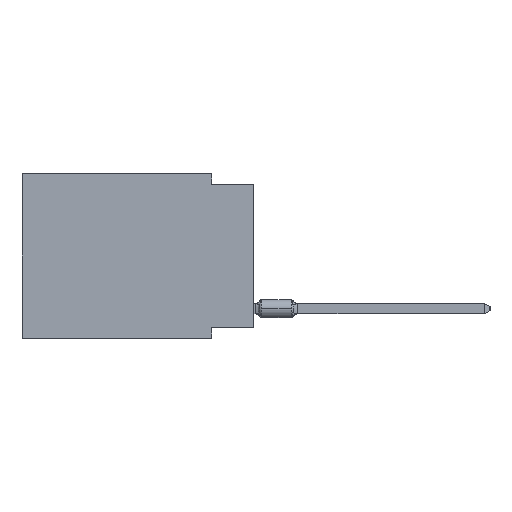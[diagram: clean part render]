
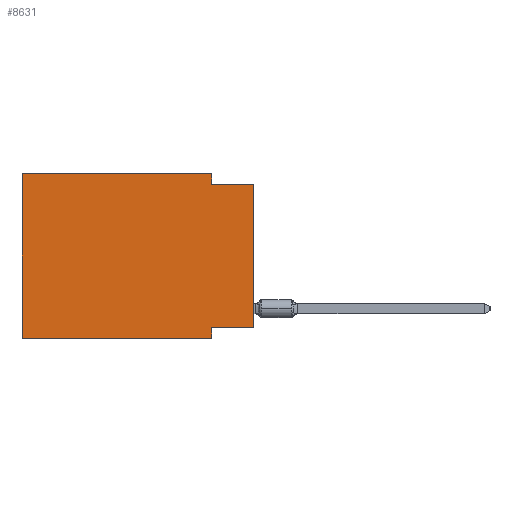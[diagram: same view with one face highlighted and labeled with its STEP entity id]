
A CAD part, left-side view. The second image highlights one B-rep face of the part: STEP entity #8631.
In plain terms, the highlighted planar face has unit normal (-1, 0, 0).
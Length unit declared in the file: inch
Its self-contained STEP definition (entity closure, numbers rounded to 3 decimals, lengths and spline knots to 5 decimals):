
#1412 = EDGE_LOOP ( 'NONE', ( #71429, #31836, #1777, #41894, #7117, #7636, #24253, #11167 ) ) ;
#1699 = DIRECTION ( 'NONE',  ( 0., -1., 0. ) ) ;
#1777 = ORIENTED_EDGE ( 'NONE', *, *, #3726, .F. ) ;
#1896 = VECTOR ( 'NONE', #9732, 39.37008 ) ;
#2048 = CARTESIAN_POINT ( 'NONE',  ( 0., 0.55, -0.39 ) ) ;
#3145 = VERTEX_POINT ( 'NONE', #2048 ) ;
#3726 = EDGE_CURVE ( 'NONE', #35269, #7681, #30704, .T. ) ;
#3989 = CARTESIAN_POINT ( 'NONE',  ( 0., 0.55, 0. ) ) ;
#7117 = ORIENTED_EDGE ( 'NONE', *, *, #74369, .F. ) ;
#7458 = CARTESIAN_POINT ( 'NONE',  ( 0., 0.55, 0. ) ) ;
#7605 = AXIS2_PLACEMENT_3D ( 'NONE', #10915, #34674, #64548 ) ;
#7636 = ORIENTED_EDGE ( 'NONE', *, *, #30221, .T. ) ;
#7681 = VERTEX_POINT ( 'NONE', #36480 ) ;
#8631 = ADVANCED_FACE ( 'NONE', ( #40813 ), #74942, .F. ) ;
#8745 = CARTESIAN_POINT ( 'NONE',  ( 0., 0.1, 0. ) ) ;
#8953 = LINE ( 'NONE', #7458, #24034 ) ;
#9732 = DIRECTION ( 'NONE',  ( 0., 0., 1. ) ) ;
#10915 = CARTESIAN_POINT ( 'NONE',  ( 0., 0.55, 0. ) ) ;
#10928 = DIRECTION ( 'NONE',  ( 0., 0., 1. ) ) ;
#11167 = ORIENTED_EDGE ( 'NONE', *, *, #50814, .F. ) ;
#11183 = EDGE_CURVE ( 'NONE', #52947, #40677, #42062, .T. ) ;
#11495 = EDGE_CURVE ( 'NONE', #67867, #63939, #34687, .T. ) ;
#13809 = LINE ( 'NONE', #54451, #18853 ) ;
#16166 = VERTEX_POINT ( 'NONE', #49203 ) ;
#17254 = VECTOR ( 'NONE', #50212, 39.37008 ) ;
#18209 = EDGE_CURVE ( 'NONE', #7681, #63939, #38442, .T. ) ;
#18433 = CARTESIAN_POINT ( 'NONE',  ( 0., 0.1, -0.39 ) ) ;
#18853 = VECTOR ( 'NONE', #67823, 39.37008 ) ;
#19587 = VECTOR ( 'NONE', #1699, 39.37008 ) ;
#23971 = VECTOR ( 'NONE', #30166, 39.37008 ) ;
#24034 = VECTOR ( 'NONE', #25063, 39.37008 ) ;
#24253 = ORIENTED_EDGE ( 'NONE', *, *, #11183, .F. ) ;
#25063 = DIRECTION ( 'NONE',  ( 0., -1., 0. ) ) ;
#28222 = DIRECTION ( 'NONE',  ( 0., 0., -1. ) ) ;
#30166 = DIRECTION ( 'NONE',  ( 0., 0., -1. ) ) ;
#30221 = EDGE_CURVE ( 'NONE', #3145, #40677, #51338, .T. ) ;
#30704 = LINE ( 'NONE', #8745, #60607 ) ;
#31836 = ORIENTED_EDGE ( 'NONE', *, *, #18209, .F. ) ;
#34674 = DIRECTION ( 'NONE',  ( 1., 0., 0. ) ) ;
#34687 = LINE ( 'NONE', #57302, #34973 ) ;
#34973 = VECTOR ( 'NONE', #10928, 39.37008 ) ;
#35269 = VERTEX_POINT ( 'NONE', #59816 ) ;
#36241 = CARTESIAN_POINT ( 'NONE',  ( 0., 0., -0.025 ) ) ;
#36480 = CARTESIAN_POINT ( 'NONE',  ( 0., 0.1, -0.025 ) ) ;
#38442 = LINE ( 'NONE', #61797, #19587 ) ;
#39613 = LINE ( 'NONE', #3989, #1896 ) ;
#40677 = VERTEX_POINT ( 'NONE', #18433 ) ;
#40813 = FACE_OUTER_BOUND ( 'NONE', #1412, .T. ) ;
#41685 = CARTESIAN_POINT ( 'NONE',  ( 0., 0.1, -0.39 ) ) ;
#41894 = ORIENTED_EDGE ( 'NONE', *, *, #55907, .F. ) ;
#42062 = LINE ( 'NONE', #41685, #23971 ) ;
#44180 = CARTESIAN_POINT ( 'NONE',  ( 0., 0.1, -0.365 ) ) ;
#44620 = CARTESIAN_POINT ( 'NONE',  ( 0., 0., -0.365 ) ) ;
#49203 = CARTESIAN_POINT ( 'NONE',  ( 0., 0.55, 0. ) ) ;
#50212 = DIRECTION ( 'NONE',  ( 0., -1., 0. ) ) ;
#50814 = EDGE_CURVE ( 'NONE', #67867, #52947, #13809, .T. ) ;
#51338 = LINE ( 'NONE', #74724, #17254 ) ;
#52947 = VERTEX_POINT ( 'NONE', #44180 ) ;
#54451 = CARTESIAN_POINT ( 'NONE',  ( 0., 0., -0.365 ) ) ;
#55907 = EDGE_CURVE ( 'NONE', #16166, #35269, #8953, .T. ) ;
#57302 = CARTESIAN_POINT ( 'NONE',  ( 0., 0., 0. ) ) ;
#59816 = CARTESIAN_POINT ( 'NONE',  ( 0., 0.1, 0. ) ) ;
#60607 = VECTOR ( 'NONE', #28222, 39.37008 ) ;
#61797 = CARTESIAN_POINT ( 'NONE',  ( 0., 0., -0.025 ) ) ;
#63939 = VERTEX_POINT ( 'NONE', #36241 ) ;
#64548 = DIRECTION ( 'NONE',  ( 0., 0., -1. ) ) ;
#67823 = DIRECTION ( 'NONE',  ( 0., 1., 0. ) ) ;
#67867 = VERTEX_POINT ( 'NONE', #44620 ) ;
#71429 = ORIENTED_EDGE ( 'NONE', *, *, #11495, .T. ) ;
#74369 = EDGE_CURVE ( 'NONE', #3145, #16166, #39613, .T. ) ;
#74724 = CARTESIAN_POINT ( 'NONE',  ( 0., 0.55, -0.39 ) ) ;
#74942 = PLANE ( 'NONE',  #7605 ) ;
